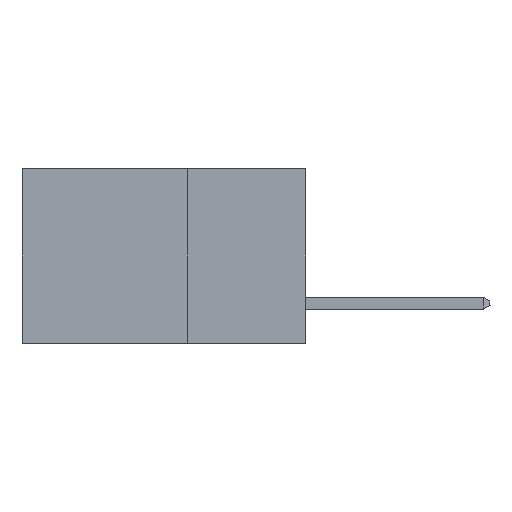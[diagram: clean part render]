
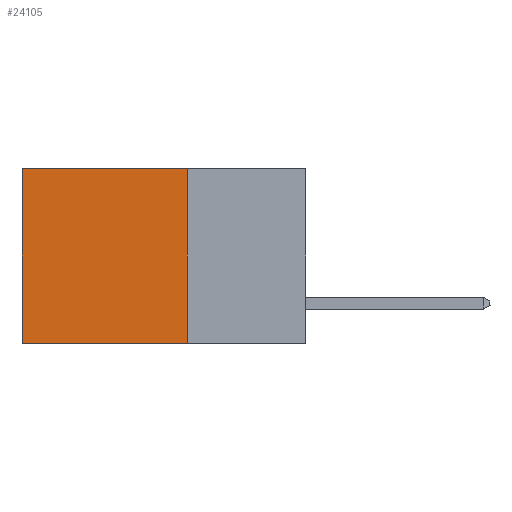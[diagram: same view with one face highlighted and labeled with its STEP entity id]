
A CAD part, left-side view. The second image highlights one B-rep face of the part: STEP entity #24105.
In plain terms, the highlighted planar face has unit normal (-1, 0, 0).
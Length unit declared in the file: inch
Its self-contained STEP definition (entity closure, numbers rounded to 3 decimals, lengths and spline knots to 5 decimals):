
#67 = CARTESIAN_POINT ( 'NONE',  ( 0.298, 0.6, 0. ) ) ;
#1426 = LINE ( 'NONE', #25996, #11281 ) ;
#3518 = VECTOR ( 'NONE', #7555, 39.37008 ) ;
#4838 = VERTEX_POINT ( 'NONE', #67 ) ;
#4997 = EDGE_CURVE ( 'NONE', #4838, #15858, #14045, .T. ) ;
#5095 = VECTOR ( 'NONE', #26305, 39.37008 ) ;
#5939 = ORIENTED_EDGE ( 'NONE', *, *, #11285, .F. ) ;
#6042 = DIRECTION ( 'NONE',  ( 0., 1., 0. ) ) ;
#6082 = LINE ( 'NONE', #23503, #16921 ) ;
#6691 = CARTESIAN_POINT ( 'NONE',  ( 0.298, 0.25, -0.37 ) ) ;
#7555 = DIRECTION ( 'NONE',  ( 0., 0., -1. ) ) ;
#8302 = CARTESIAN_POINT ( 'NONE',  ( 0.298, 0.6, -0.37 ) ) ;
#8390 = VERTEX_POINT ( 'NONE', #6691 ) ;
#11086 = ORIENTED_EDGE ( 'NONE', *, *, #4997, .T. ) ;
#11109 = CARTESIAN_POINT ( 'NONE',  ( 0.298, 0.25, -0.37 ) ) ;
#11281 = VECTOR ( 'NONE', #20224, 39.37008 ) ;
#11285 = EDGE_CURVE ( 'NONE', #8390, #15858, #22740, .T. ) ;
#13361 = CARTESIAN_POINT ( 'NONE',  ( 0.298, 0.6, 0. ) ) ;
#13594 = ORIENTED_EDGE ( 'NONE', *, *, #20363, .T. ) ;
#14045 = LINE ( 'NONE', #13361, #3518 ) ;
#14718 = EDGE_CURVE ( 'NONE', #24173, #8390, #1426, .T. ) ;
#15271 = CARTESIAN_POINT ( 'NONE',  ( 0.298, 0.25, 0. ) ) ;
#15719 = AXIS2_PLACEMENT_3D ( 'NONE', #15271, #27994, #26207 ) ;
#15858 = VERTEX_POINT ( 'NONE', #8302 ) ;
#16921 = VECTOR ( 'NONE', #6042, 39.37008 ) ;
#20224 = DIRECTION ( 'NONE',  ( 0., 0., -1. ) ) ;
#20363 = EDGE_CURVE ( 'NONE', #24173, #4838, #6082, .T. ) ;
#20442 = EDGE_LOOP ( 'NONE', ( #11086, #5939, #27730, #13594 ) ) ;
#22740 = LINE ( 'NONE', #11109, #5095 ) ;
#23503 = CARTESIAN_POINT ( 'NONE',  ( 0.298, 0.25, 0. ) ) ;
#24105 = ADVANCED_FACE ( 'NONE', ( #24972 ), #25820, .F. ) ;
#24173 = VERTEX_POINT ( 'NONE', #25911 ) ;
#24972 = FACE_OUTER_BOUND ( 'NONE', #20442, .T. ) ;
#25820 = PLANE ( 'NONE',  #15719 ) ;
#25911 = CARTESIAN_POINT ( 'NONE',  ( 0.298, 0.25, 0. ) ) ;
#25996 = CARTESIAN_POINT ( 'NONE',  ( 0.298, 0.25, 0. ) ) ;
#26207 = DIRECTION ( 'NONE',  ( 0., 0., -1. ) ) ;
#26305 = DIRECTION ( 'NONE',  ( 0., 1., 0. ) ) ;
#27730 = ORIENTED_EDGE ( 'NONE', *, *, #14718, .F. ) ;
#27994 = DIRECTION ( 'NONE',  ( 1., 0., 0. ) ) ;
